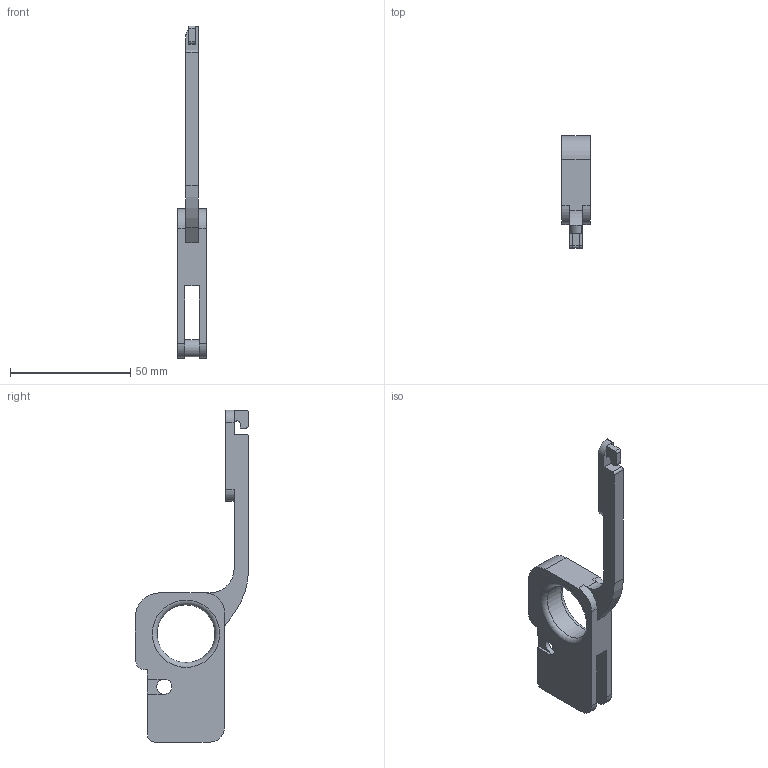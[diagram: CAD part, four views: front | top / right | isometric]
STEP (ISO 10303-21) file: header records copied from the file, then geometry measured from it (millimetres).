
FILE_DESCRIPTION((''),'2;1');
FILE_NAME('PM522Trigger2.stp','2015-10-01T18:16:44',('JamesRPatrick'),(''),'Autodesk Inventor 2012','Autodesk Inventor 2012','');
FILE_SCHEMA(('AUTOMOTIVE_DESIGN { 1 0 10303 214 1 1 1 1 }'));
Length unit declared in the file: millimetre
Products named in the file (1): PM522Trigger2
Bounding box: 12 x 47 x 138 mm (x, y, z)
Volume: 17332.2 mm3; surface area: 10156.7 mm2
Topology: 1 solids, 1 shells, 54 faces, 155 edges, 102 vertices
Faces by surface type: plane 32, cylinder 20, torus 2
Full cylindrical faces by diameter (mm): 6.2 x2, 7 x1, 24 x1
Entity records: 1775 total; most frequent: CARTESIAN_POINT 304, DIRECTION 303, ORIENTED_EDGE 296, EDGE_CURVE 148, VECTOR 103, LINE 103, VERTEX_POINT 101, AXIS2_PLACEMENT_3D 100
